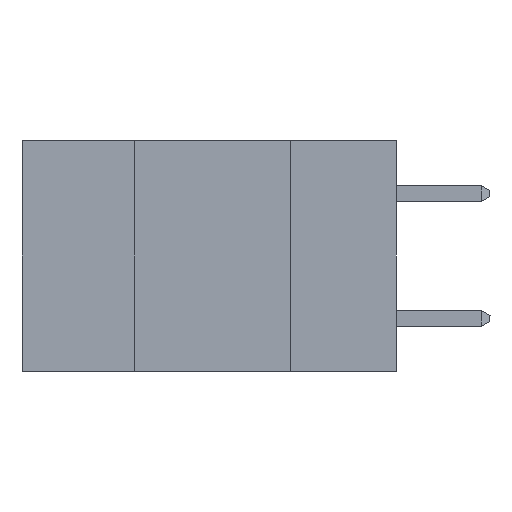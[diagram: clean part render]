
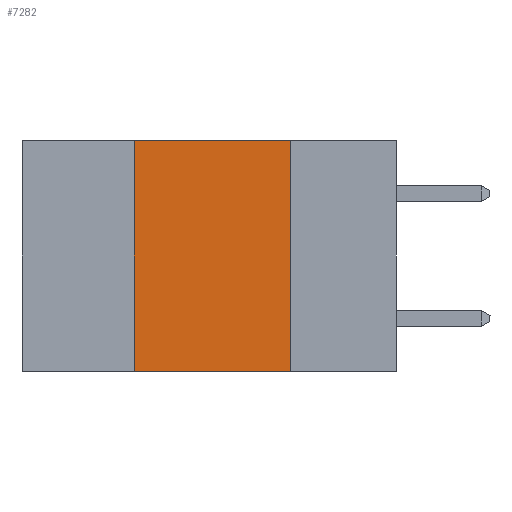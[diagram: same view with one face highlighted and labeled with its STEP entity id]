
A CAD part, left-side view. The second image highlights one B-rep face of the part: STEP entity #7282.
In plain terms, the highlighted planar face has unit normal (-1, 0, 0).
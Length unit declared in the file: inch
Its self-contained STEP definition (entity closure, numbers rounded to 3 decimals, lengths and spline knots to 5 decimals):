
#1238 = CARTESIAN_POINT ( 'NONE',  ( 0., 0.17, -0.37 ) ) ;
#2416 = LINE ( 'NONE', #12717, #13662 ) ;
#2803 = EDGE_CURVE ( 'NONE', #3223, #14695, #8475, .T. ) ;
#2940 = CARTESIAN_POINT ( 'NONE',  ( 0., 0.17, 0. ) ) ;
#3135 = VECTOR ( 'NONE', #4878, 39.37008 ) ;
#3223 = VERTEX_POINT ( 'NONE', #10484 ) ;
#3902 = LINE ( 'NONE', #8037, #6734 ) ;
#4637 = FACE_OUTER_BOUND ( 'NONE', #18049, .T. ) ;
#4878 = DIRECTION ( 'NONE',  ( 0., -1., 0. ) ) ;
#5052 = CARTESIAN_POINT ( 'NONE',  ( 0., 0.6, 0. ) ) ;
#5349 = ORIENTED_EDGE ( 'NONE', *, *, #18242, .T. ) ;
#5647 = EDGE_CURVE ( 'NONE', #14695, #7764, #10108, .T. ) ;
#5665 = VECTOR ( 'NONE', #16456, 39.37008 ) ;
#6575 = EDGE_CURVE ( 'NONE', #7764, #17468, #2416, .T. ) ;
#6734 = VECTOR ( 'NONE', #15163, 39.37008 ) ;
#6792 = DIRECTION ( 'NONE',  ( 0., 0., -1. ) ) ;
#6809 = DIRECTION ( 'NONE',  ( 1., 0., 0. ) ) ;
#6870 = PLANE ( 'NONE',  #9529 ) ;
#6931 = CARTESIAN_POINT ( 'NONE',  ( 0., 0.6, 0. ) ) ;
#7282 = ADVANCED_FACE ( 'NONE', ( #4637 ), #6870, .F. ) ;
#7697 = ORIENTED_EDGE ( 'NONE', *, *, #6575, .F. ) ;
#7764 = VERTEX_POINT ( 'NONE', #2940 ) ;
#8037 = CARTESIAN_POINT ( 'NONE',  ( 0., 0.6, -0.37 ) ) ;
#8475 = LINE ( 'NONE', #9008, #5665 ) ;
#9008 = CARTESIAN_POINT ( 'NONE',  ( 0., 0.42, -0.37 ) ) ;
#9529 = AXIS2_PLACEMENT_3D ( 'NONE', #6931, #6809, #6792 ) ;
#10108 = LINE ( 'NONE', #5052, #3135 ) ;
#10484 = CARTESIAN_POINT ( 'NONE',  ( 0., 0.42, -0.37 ) ) ;
#12126 = CARTESIAN_POINT ( 'NONE',  ( 0., 0.42, 0. ) ) ;
#12341 = ORIENTED_EDGE ( 'NONE', *, *, #2803, .F. ) ;
#12691 = DIRECTION ( 'NONE',  ( 0., 0., -1. ) ) ;
#12717 = CARTESIAN_POINT ( 'NONE',  ( 0., 0.17, -0.37 ) ) ;
#13662 = VECTOR ( 'NONE', #12691, 39.37008 ) ;
#14695 = VERTEX_POINT ( 'NONE', #12126 ) ;
#15163 = DIRECTION ( 'NONE',  ( 0., -1., 0. ) ) ;
#15253 = ORIENTED_EDGE ( 'NONE', *, *, #5647, .F. ) ;
#16456 = DIRECTION ( 'NONE',  ( 0., 0., 1. ) ) ;
#17468 = VERTEX_POINT ( 'NONE', #1238 ) ;
#18049 = EDGE_LOOP ( 'NONE', ( #7697, #15253, #12341, #5349 ) ) ;
#18242 = EDGE_CURVE ( 'NONE', #3223, #17468, #3902, .T. ) ;
